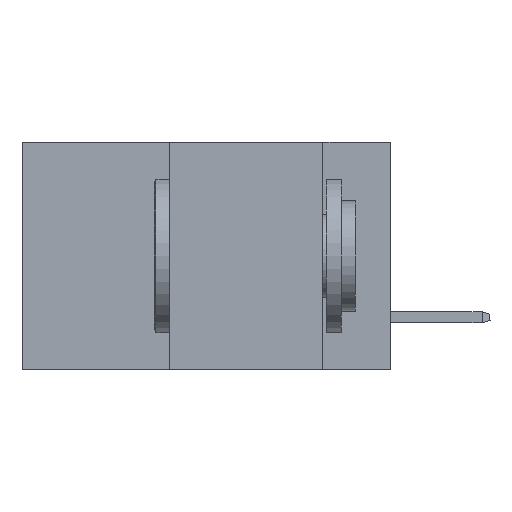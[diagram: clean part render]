
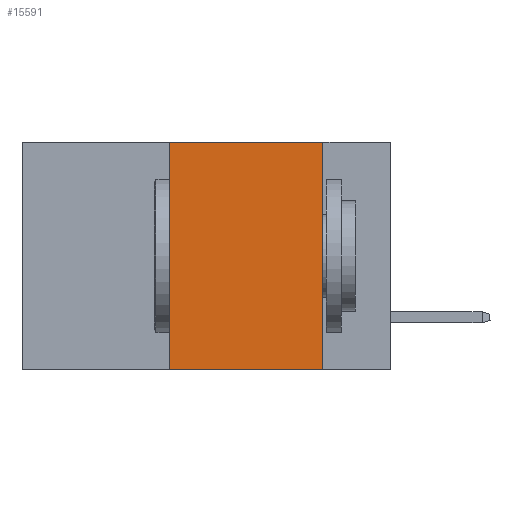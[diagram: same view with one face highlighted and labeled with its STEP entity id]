
A CAD part, left-side view. The second image highlights one B-rep face of the part: STEP entity #15591.
In plain terms, the highlighted planar face has unit normal (-1, 0, 0).
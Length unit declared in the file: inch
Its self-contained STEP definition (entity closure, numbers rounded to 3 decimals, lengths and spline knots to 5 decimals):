
#915 = VECTOR ( 'NONE', #3048, 39.37008 ) ;
#1055 = EDGE_LOOP ( 'NONE', ( #9557, #1121, #15882, #4730 ) ) ;
#1121 = ORIENTED_EDGE ( 'NONE', *, *, #15051, .F. ) ;
#1163 = VECTOR ( 'NONE', #2751, 39.37008 ) ;
#1306 = EDGE_CURVE ( 'NONE', #13496, #15597, #1362, .T. ) ;
#1362 = LINE ( 'NONE', #7607, #1163 ) ;
#1467 = AXIS2_PLACEMENT_3D ( 'NONE', #12494, #11580, #5391 ) ;
#1946 = VERTEX_POINT ( 'NONE', #5564 ) ;
#2071 = LINE ( 'NONE', #11884, #915 ) ;
#2585 = LINE ( 'NONE', #9948, #15690 ) ;
#2751 = DIRECTION ( 'NONE',  ( 0., -1., 0. ) ) ;
#3048 = DIRECTION ( 'NONE',  ( 0., -1., 0. ) ) ;
#4730 = ORIENTED_EDGE ( 'NONE', *, *, #1306, .T. ) ;
#4876 = DIRECTION ( 'NONE',  ( 0., 0., 1. ) ) ;
#4893 = CARTESIAN_POINT ( 'NONE',  ( 0., 0.11, 0. ) ) ;
#4991 = EDGE_CURVE ( 'NONE', #13496, #1946, #2585, .T. ) ;
#5391 = DIRECTION ( 'NONE',  ( 0., 0., -1. ) ) ;
#5564 = CARTESIAN_POINT ( 'NONE',  ( 0., 0.36, 0. ) ) ;
#6659 = VECTOR ( 'NONE', #7579, 39.37008 ) ;
#6859 = CARTESIAN_POINT ( 'NONE',  ( 0., 0.11, 0. ) ) ;
#7579 = DIRECTION ( 'NONE',  ( 0., 0., -1. ) ) ;
#7607 = CARTESIAN_POINT ( 'NONE',  ( 0., 0.6, -0.37 ) ) ;
#9557 = ORIENTED_EDGE ( 'NONE', *, *, #11856, .F. ) ;
#9948 = CARTESIAN_POINT ( 'NONE',  ( 0., 0.36, 0. ) ) ;
#11580 = DIRECTION ( 'NONE',  ( 1., 0., 0. ) ) ;
#11785 = PLANE ( 'NONE',  #1467 ) ;
#11856 = EDGE_CURVE ( 'NONE', #12048, #15597, #13834, .T. ) ;
#11884 = CARTESIAN_POINT ( 'NONE',  ( 0., 0.6, 0. ) ) ;
#12048 = VERTEX_POINT ( 'NONE', #6859 ) ;
#12494 = CARTESIAN_POINT ( 'NONE',  ( 0., 0.6, 0. ) ) ;
#12512 = CARTESIAN_POINT ( 'NONE',  ( 0., 0.11, -0.37 ) ) ;
#13496 = VERTEX_POINT ( 'NONE', #13565 ) ;
#13565 = CARTESIAN_POINT ( 'NONE',  ( 0., 0.36, -0.37 ) ) ;
#13834 = LINE ( 'NONE', #4893, #6659 ) ;
#15051 = EDGE_CURVE ( 'NONE', #1946, #12048, #2071, .T. ) ;
#15380 = FACE_OUTER_BOUND ( 'NONE', #1055, .T. ) ;
#15591 = ADVANCED_FACE ( 'NONE', ( #15380 ), #11785, .F. ) ;
#15597 = VERTEX_POINT ( 'NONE', #12512 ) ;
#15690 = VECTOR ( 'NONE', #4876, 39.37008 ) ;
#15882 = ORIENTED_EDGE ( 'NONE', *, *, #4991, .F. ) ;
